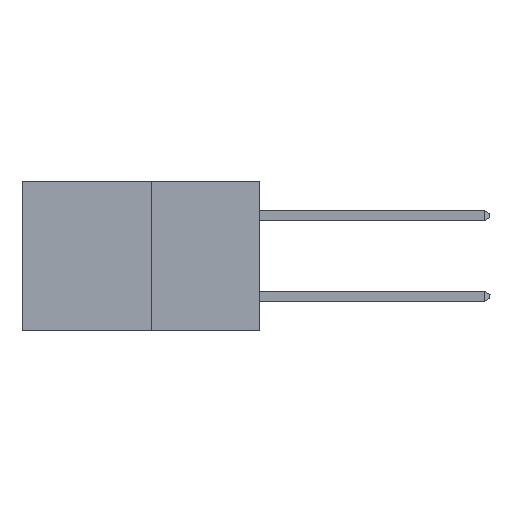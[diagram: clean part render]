
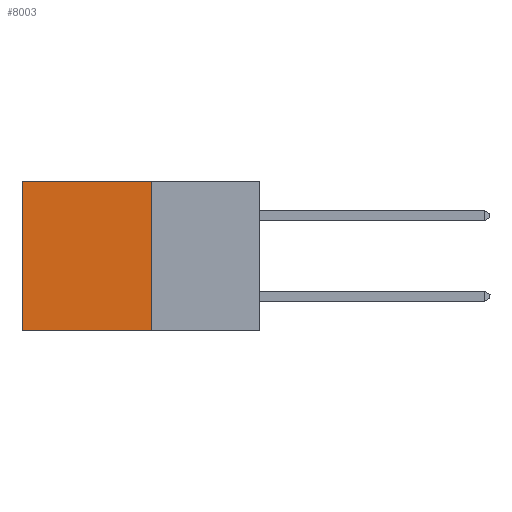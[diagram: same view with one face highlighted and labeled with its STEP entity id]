
A CAD part, left-side view. The second image highlights one B-rep face of the part: STEP entity #8003.
In plain terms, the highlighted planar face has unit normal (-1, 0, 0).
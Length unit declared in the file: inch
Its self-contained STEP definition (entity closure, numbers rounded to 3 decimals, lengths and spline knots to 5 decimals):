
#196 = ORIENTED_EDGE ( 'NONE', *, *, #15568, .T. ) ;
#220 = EDGE_CURVE ( 'NONE', #4064, #4837, #2917, .T. ) ;
#445 = ORIENTED_EDGE ( 'NONE', *, *, #7363, .F. ) ;
#979 = DIRECTION ( 'NONE',  ( 0., 0., -1. ) ) ;
#1140 = VERTEX_POINT ( 'NONE', #12927 ) ;
#1461 = CARTESIAN_POINT ( 'NONE',  ( 0.277, 0.27, -0.37 ) ) ;
#2917 = LINE ( 'NONE', #18675, #15605 ) ;
#4064 = VERTEX_POINT ( 'NONE', #14158 ) ;
#4837 = VERTEX_POINT ( 'NONE', #1461 ) ;
#5333 = VERTEX_POINT ( 'NONE', #13894 ) ;
#5709 = LINE ( 'NONE', #11004, #9590 ) ;
#6150 = DIRECTION ( 'NONE',  ( 0., 0., -1. ) ) ;
#6208 = ORIENTED_EDGE ( 'NONE', *, *, #20107, .T. ) ;
#6797 = FACE_OUTER_BOUND ( 'NONE', #20173, .T. ) ;
#7363 = EDGE_CURVE ( 'NONE', #4837, #1140, #14740, .T. ) ;
#8003 = ADVANCED_FACE ( 'NONE', ( #6797 ), #10589, .F. ) ;
#9590 = VECTOR ( 'NONE', #16006, 39.37008 ) ;
#10514 = DIRECTION ( 'NONE',  ( 0., 0., -1. ) ) ;
#10555 = DIRECTION ( 'NONE',  ( 1., 0., 0. ) ) ;
#10589 = PLANE ( 'NONE',  #13508 ) ;
#10682 = CARTESIAN_POINT ( 'NONE',  ( 0.277, 0.27, -0.37 ) ) ;
#11004 = CARTESIAN_POINT ( 'NONE',  ( 0.277, 0.27, 0. ) ) ;
#11930 = VECTOR ( 'NONE', #979, 39.37008 ) ;
#12437 = LINE ( 'NONE', #20765, #11930 ) ;
#12927 = CARTESIAN_POINT ( 'NONE',  ( 0.277, 0.59, -0.37 ) ) ;
#13508 = AXIS2_PLACEMENT_3D ( 'NONE', #10682, #10555, #10514 ) ;
#13894 = CARTESIAN_POINT ( 'NONE',  ( 0.277, 0.59, 0. ) ) ;
#14158 = CARTESIAN_POINT ( 'NONE',  ( 0.277, 0.27, 0. ) ) ;
#14218 = VECTOR ( 'NONE', #16334, 39.37008 ) ;
#14740 = LINE ( 'NONE', #16315, #14218 ) ;
#15568 = EDGE_CURVE ( 'NONE', #4064, #5333, #5709, .T. ) ;
#15605 = VECTOR ( 'NONE', #6150, 39.37008 ) ;
#16006 = DIRECTION ( 'NONE',  ( 0., 1., 0. ) ) ;
#16315 = CARTESIAN_POINT ( 'NONE',  ( 0.277, 0.27, -0.37 ) ) ;
#16334 = DIRECTION ( 'NONE',  ( 0., 1., 0. ) ) ;
#18675 = CARTESIAN_POINT ( 'NONE',  ( 0.277, 0.27, -0.37 ) ) ;
#20107 = EDGE_CURVE ( 'NONE', #5333, #1140, #12437, .T. ) ;
#20173 = EDGE_LOOP ( 'NONE', ( #6208, #445, #21155, #196 ) ) ;
#20765 = CARTESIAN_POINT ( 'NONE',  ( 0.277, 0.59, -0.37 ) ) ;
#21155 = ORIENTED_EDGE ( 'NONE', *, *, #220, .F. ) ;
